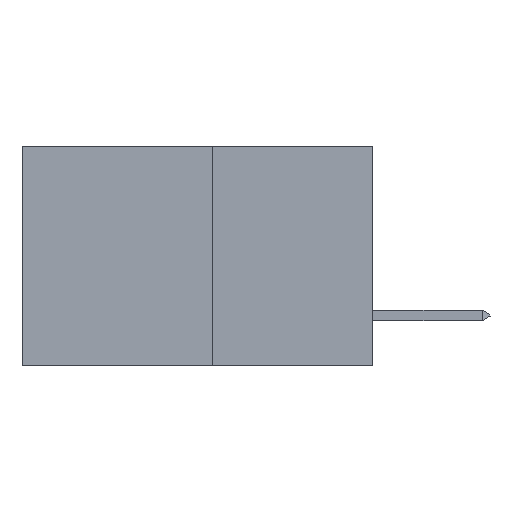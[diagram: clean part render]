
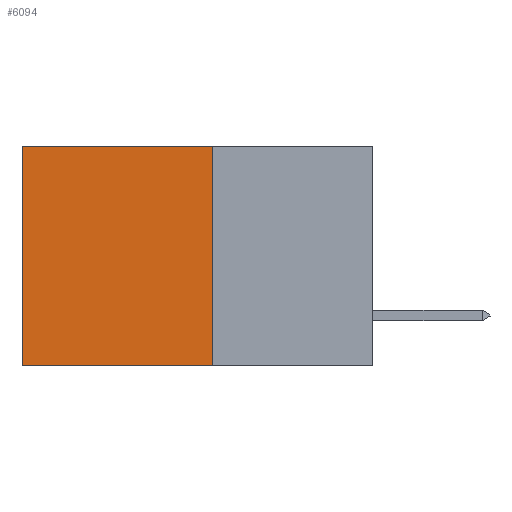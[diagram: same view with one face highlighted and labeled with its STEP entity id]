
A CAD part, left-side view. The second image highlights one B-rep face of the part: STEP entity #6094.
In plain terms, the highlighted planar face has unit normal (-1, 0, 0).
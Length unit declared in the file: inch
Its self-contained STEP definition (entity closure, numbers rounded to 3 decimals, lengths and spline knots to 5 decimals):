
#914 = VERTEX_POINT ( 'NONE', #13432 ) ;
#1056 = VECTOR ( 'NONE', #10060, 39.37008 ) ;
#1823 = CARTESIAN_POINT ( 'NONE',  ( 0.277, 0.27, -0.37 ) ) ;
#2234 = DIRECTION ( 'NONE',  ( 0., 0., -1. ) ) ;
#2711 = EDGE_CURVE ( 'NONE', #7135, #3282, #14126, .T. ) ;
#2725 = DIRECTION ( 'NONE',  ( 0., 1., 0. ) ) ;
#3106 = CARTESIAN_POINT ( 'NONE',  ( 0.277, 0.27, 0. ) ) ;
#3282 = VERTEX_POINT ( 'NONE', #3984 ) ;
#3318 = EDGE_CURVE ( 'NONE', #7135, #7159, #12347, .T. ) ;
#3984 = CARTESIAN_POINT ( 'NONE',  ( 0.277, 0.27, -0.37 ) ) ;
#4557 = FACE_OUTER_BOUND ( 'NONE', #9036, .T. ) ;
#4736 = ORIENTED_EDGE ( 'NONE', *, *, #3318, .T. ) ;
#5124 = EDGE_CURVE ( 'NONE', #3282, #914, #8727, .T. ) ;
#5541 = VECTOR ( 'NONE', #2725, 39.37008 ) ;
#5850 = ORIENTED_EDGE ( 'NONE', *, *, #2711, .F. ) ;
#6094 = ADVANCED_FACE ( 'NONE', ( #4557 ), #13219, .F. ) ;
#6118 = VECTOR ( 'NONE', #10169, 39.37008 ) ;
#7129 = ORIENTED_EDGE ( 'NONE', *, *, #8348, .T. ) ;
#7135 = VERTEX_POINT ( 'NONE', #10106 ) ;
#7144 = ORIENTED_EDGE ( 'NONE', *, *, #5124, .F. ) ;
#7159 = VERTEX_POINT ( 'NONE', #10842 ) ;
#8344 = CARTESIAN_POINT ( 'NONE',  ( 0.277, 0.59, -0.37 ) ) ;
#8348 = EDGE_CURVE ( 'NONE', #7159, #914, #10050, .T. ) ;
#8727 = LINE ( 'NONE', #1823, #5541 ) ;
#9036 = EDGE_LOOP ( 'NONE', ( #7129, #7144, #5850, #4736 ) ) ;
#9412 = DIRECTION ( 'NONE',  ( 0., 0., -1. ) ) ;
#10050 = LINE ( 'NONE', #8344, #12768 ) ;
#10060 = DIRECTION ( 'NONE',  ( 0., 0., -1. ) ) ;
#10106 = CARTESIAN_POINT ( 'NONE',  ( 0.277, 0.27, 0. ) ) ;
#10169 = DIRECTION ( 'NONE',  ( 0., 1., 0. ) ) ;
#10842 = CARTESIAN_POINT ( 'NONE',  ( 0.277, 0.59, 0. ) ) ;
#12347 = LINE ( 'NONE', #3106, #6118 ) ;
#12768 = VECTOR ( 'NONE', #2234, 39.37008 ) ;
#12825 = DIRECTION ( 'NONE',  ( 1., 0., 0. ) ) ;
#12863 = CARTESIAN_POINT ( 'NONE',  ( 0.277, 0.27, -0.37 ) ) ;
#13219 = PLANE ( 'NONE',  #14052 ) ;
#13432 = CARTESIAN_POINT ( 'NONE',  ( 0.277, 0.59, -0.37 ) ) ;
#14052 = AXIS2_PLACEMENT_3D ( 'NONE', #12863, #12825, #9412 ) ;
#14126 = LINE ( 'NONE', #14687, #1056 ) ;
#14687 = CARTESIAN_POINT ( 'NONE',  ( 0.277, 0.27, -0.37 ) ) ;
